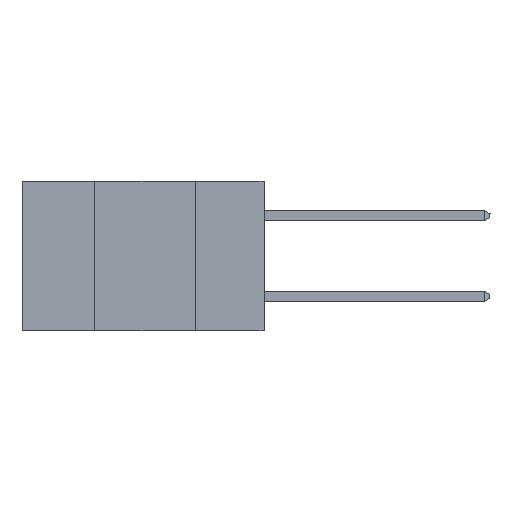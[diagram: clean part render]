
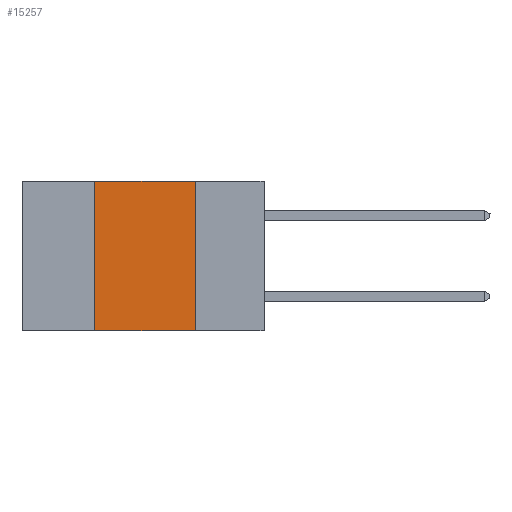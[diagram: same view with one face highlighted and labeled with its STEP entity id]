
A CAD part, left-side view. The second image highlights one B-rep face of the part: STEP entity #15257.
In plain terms, the highlighted planar face has unit normal (-1, 0, 0).
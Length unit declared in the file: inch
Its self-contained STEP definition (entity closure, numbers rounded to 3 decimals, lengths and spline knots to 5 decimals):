
#245 = CARTESIAN_POINT ( 'NONE',  ( 0., 0.6, -0.37 ) ) ;
#544 = ORIENTED_EDGE ( 'NONE', *, *, #4528, .F. ) ;
#691 = EDGE_CURVE ( 'NONE', #2687, #4470, #24417, .T. ) ;
#771 = CARTESIAN_POINT ( 'NONE',  ( 0., 0.6, 0. ) ) ;
#2687 = VERTEX_POINT ( 'NONE', #9397 ) ;
#2967 = CARTESIAN_POINT ( 'NONE',  ( 0., 0.6, 0. ) ) ;
#3623 = ORIENTED_EDGE ( 'NONE', *, *, #691, .T. ) ;
#4132 = EDGE_CURVE ( 'NONE', #2687, #5992, #18658, .T. ) ;
#4470 = VERTEX_POINT ( 'NONE', #16785 ) ;
#4528 = EDGE_CURVE ( 'NONE', #27539, #4470, #9721, .T. ) ;
#4649 = VECTOR ( 'NONE', #26734, 39.37008 ) ;
#4882 = VECTOR ( 'NONE', #15133, 39.37008 ) ;
#5468 = PLANE ( 'NONE',  #13957 ) ;
#5992 = VERTEX_POINT ( 'NONE', #11231 ) ;
#7005 = EDGE_CURVE ( 'NONE', #5992, #27539, #27719, .T. ) ;
#7457 = CARTESIAN_POINT ( 'NONE',  ( 0., 0.17, 0. ) ) ;
#9397 = CARTESIAN_POINT ( 'NONE',  ( 0., 0.42, -0.37 ) ) ;
#9721 = LINE ( 'NONE', #7457, #19728 ) ;
#9727 = FACE_OUTER_BOUND ( 'NONE', #23496, .T. ) ;
#10349 = CARTESIAN_POINT ( 'NONE',  ( 0., 0.42, 0. ) ) ;
#11231 = CARTESIAN_POINT ( 'NONE',  ( 0., 0.42, 0. ) ) ;
#13957 = AXIS2_PLACEMENT_3D ( 'NONE', #771, #17426, #24109 ) ;
#15133 = DIRECTION ( 'NONE',  ( 0., 0., 1. ) ) ;
#15257 = ADVANCED_FACE ( 'NONE', ( #9727 ), #5468, .F. ) ;
#16052 = ORIENTED_EDGE ( 'NONE', *, *, #7005, .F. ) ;
#16785 = CARTESIAN_POINT ( 'NONE',  ( 0., 0.17, -0.37 ) ) ;
#17185 = DIRECTION ( 'NONE',  ( 0., 0., -1. ) ) ;
#17426 = DIRECTION ( 'NONE',  ( 1., 0., 0. ) ) ;
#18658 = LINE ( 'NONE', #10349, #4882 ) ;
#19728 = VECTOR ( 'NONE', #17185, 39.37008 ) ;
#22726 = CARTESIAN_POINT ( 'NONE',  ( 0., 0.17, 0. ) ) ;
#23496 = EDGE_LOOP ( 'NONE', ( #544, #16052, #23507, #3623 ) ) ;
#23507 = ORIENTED_EDGE ( 'NONE', *, *, #4132, .F. ) ;
#24109 = DIRECTION ( 'NONE',  ( 0., 0., -1. ) ) ;
#24417 = LINE ( 'NONE', #245, #25531 ) ;
#25531 = VECTOR ( 'NONE', #29731, 39.37008 ) ;
#26734 = DIRECTION ( 'NONE',  ( 0., -1., 0. ) ) ;
#27539 = VERTEX_POINT ( 'NONE', #22726 ) ;
#27719 = LINE ( 'NONE', #2967, #4649 ) ;
#29731 = DIRECTION ( 'NONE',  ( 0., -1., 0. ) ) ;
